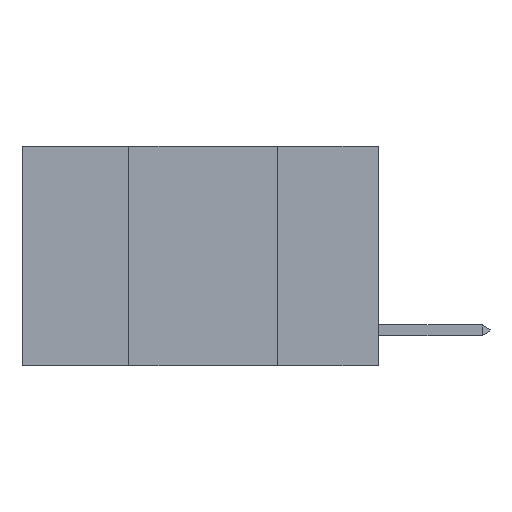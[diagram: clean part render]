
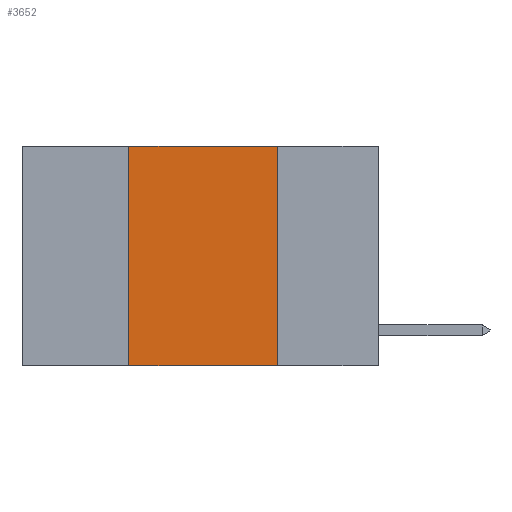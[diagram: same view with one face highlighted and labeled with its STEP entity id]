
A CAD part, left-side view. The second image highlights one B-rep face of the part: STEP entity #3652.
In plain terms, the highlighted planar face has unit normal (-1, 0, 0).
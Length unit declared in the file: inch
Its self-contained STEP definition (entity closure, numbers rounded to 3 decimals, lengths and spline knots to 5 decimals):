
#44 = DIRECTION ( 'NONE',  ( 0., -1., 0. ) ) ;
#718 = CARTESIAN_POINT ( 'NONE',  ( 0., 0.17, -0.37 ) ) ;
#776 = LINE ( 'NONE', #7963, #11416 ) ;
#862 = ORIENTED_EDGE ( 'NONE', *, *, #7613, .F. ) ;
#940 = EDGE_LOOP ( 'NONE', ( #6043, #862, #11290, #9341 ) ) ;
#1359 = CARTESIAN_POINT ( 'NONE',  ( 0., 0.6, 0. ) ) ;
#1579 = CARTESIAN_POINT ( 'NONE',  ( 0., 0.42, -0.37 ) ) ;
#1608 = DIRECTION ( 'NONE',  ( 0., 0., -1. ) ) ;
#2259 = DIRECTION ( 'NONE',  ( 0., 0., -1. ) ) ;
#2300 = CARTESIAN_POINT ( 'NONE',  ( 0., 0.6, 0. ) ) ;
#2673 = CARTESIAN_POINT ( 'NONE',  ( 0., 0.17, 0. ) ) ;
#2771 = AXIS2_PLACEMENT_3D ( 'NONE', #2300, #5438, #1608 ) ;
#3633 = PLANE ( 'NONE',  #2771 ) ;
#3652 = ADVANCED_FACE ( 'NONE', ( #13112 ), #3633, .F. ) ;
#4341 = EDGE_CURVE ( 'NONE', #12659, #12792, #6450, .T. ) ;
#4777 = DIRECTION ( 'NONE',  ( 0., 0., 1. ) ) ;
#4967 = EDGE_CURVE ( 'NONE', #6209, #12792, #5019, .T. ) ;
#5019 = LINE ( 'NONE', #12322, #7581 ) ;
#5438 = DIRECTION ( 'NONE',  ( 1., 0., 0. ) ) ;
#6043 = ORIENTED_EDGE ( 'NONE', *, *, #4341, .F. ) ;
#6107 = VECTOR ( 'NONE', #2259, 39.37008 ) ;
#6209 = VERTEX_POINT ( 'NONE', #1579 ) ;
#6255 = CARTESIAN_POINT ( 'NONE',  ( 0., 0.42, 0. ) ) ;
#6450 = LINE ( 'NONE', #9584, #6107 ) ;
#7581 = VECTOR ( 'NONE', #44, 39.37008 ) ;
#7613 = EDGE_CURVE ( 'NONE', #10137, #12659, #12179, .T. ) ;
#7963 = CARTESIAN_POINT ( 'NONE',  ( 0., 0.42, 0. ) ) ;
#9341 = ORIENTED_EDGE ( 'NONE', *, *, #4967, .T. ) ;
#9371 = VECTOR ( 'NONE', #11624, 39.37008 ) ;
#9584 = CARTESIAN_POINT ( 'NONE',  ( 0., 0.17, 0. ) ) ;
#10137 = VERTEX_POINT ( 'NONE', #6255 ) ;
#10740 = EDGE_CURVE ( 'NONE', #6209, #10137, #776, .T. ) ;
#11290 = ORIENTED_EDGE ( 'NONE', *, *, #10740, .F. ) ;
#11416 = VECTOR ( 'NONE', #4777, 39.37008 ) ;
#11624 = DIRECTION ( 'NONE',  ( 0., -1., 0. ) ) ;
#12179 = LINE ( 'NONE', #1359, #9371 ) ;
#12322 = CARTESIAN_POINT ( 'NONE',  ( 0., 0.6, -0.37 ) ) ;
#12659 = VERTEX_POINT ( 'NONE', #2673 ) ;
#12792 = VERTEX_POINT ( 'NONE', #718 ) ;
#13112 = FACE_OUTER_BOUND ( 'NONE', #940, .T. ) ;
